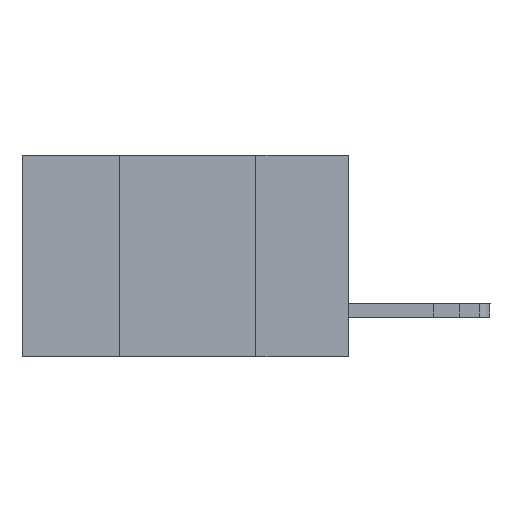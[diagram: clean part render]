
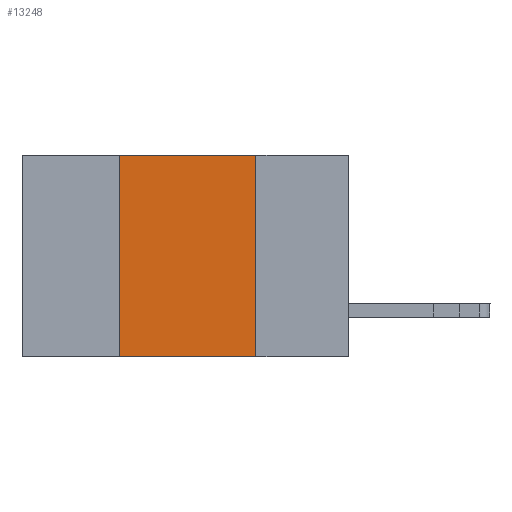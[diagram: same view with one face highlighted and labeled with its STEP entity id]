
A CAD part, left-side view. The second image highlights one B-rep face of the part: STEP entity #13248.
In plain terms, the highlighted planar face has unit normal (-1, 0, 0).
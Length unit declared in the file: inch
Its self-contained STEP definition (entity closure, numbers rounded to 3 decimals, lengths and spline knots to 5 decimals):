
#283 = VECTOR ( 'NONE', #841, 39.37008 ) ;
#434 = CARTESIAN_POINT ( 'NONE',  ( 0., 0.6, -0.37 ) ) ;
#621 = AXIS2_PLACEMENT_3D ( 'NONE', #13764, #3390, #15486 ) ;
#841 = DIRECTION ( 'NONE',  ( 0., -1., 0. ) ) ;
#1753 = VERTEX_POINT ( 'NONE', #9347 ) ;
#1844 = ORIENTED_EDGE ( 'NONE', *, *, #4746, .T. ) ;
#1912 = ORIENTED_EDGE ( 'NONE', *, *, #3890, .F. ) ;
#1971 = CARTESIAN_POINT ( 'NONE',  ( 0., 0.17, -0.37 ) ) ;
#3390 = DIRECTION ( 'NONE',  ( 1., 0., 0. ) ) ;
#3890 = EDGE_CURVE ( 'NONE', #1753, #20682, #10114, .T. ) ;
#4715 = ORIENTED_EDGE ( 'NONE', *, *, #16587, .F. ) ;
#4746 = EDGE_CURVE ( 'NONE', #8579, #16002, #18567, .T. ) ;
#5558 = LINE ( 'NONE', #10077, #14237 ) ;
#5957 = CARTESIAN_POINT ( 'NONE',  ( 0., 0.17, 0. ) ) ;
#8068 = EDGE_LOOP ( 'NONE', ( #4715, #1912, #21949, #1844 ) ) ;
#8579 = VERTEX_POINT ( 'NONE', #21644 ) ;
#9347 = CARTESIAN_POINT ( 'NONE',  ( 0., 0.42, 0. ) ) ;
#10077 = CARTESIAN_POINT ( 'NONE',  ( 0., 0.42, -0.37 ) ) ;
#10114 = LINE ( 'NONE', #14477, #14135 ) ;
#10313 = PLANE ( 'NONE',  #621 ) ;
#11211 = FACE_OUTER_BOUND ( 'NONE', #8068, .T. ) ;
#12227 = CARTESIAN_POINT ( 'NONE',  ( 0., 0.17, -0.37 ) ) ;
#13248 = ADVANCED_FACE ( 'NONE', ( #11211 ), #10313, .F. ) ;
#13764 = CARTESIAN_POINT ( 'NONE',  ( 0., 0.6, 0. ) ) ;
#13959 = DIRECTION ( 'NONE',  ( 0., -1., 0. ) ) ;
#14135 = VECTOR ( 'NONE', #13959, 39.37008 ) ;
#14237 = VECTOR ( 'NONE', #21908, 39.37008 ) ;
#14477 = CARTESIAN_POINT ( 'NONE',  ( 0., 0.6, 0. ) ) ;
#15486 = DIRECTION ( 'NONE',  ( 0., 0., -1. ) ) ;
#16002 = VERTEX_POINT ( 'NONE', #1971 ) ;
#16587 = EDGE_CURVE ( 'NONE', #20682, #16002, #21035, .T. ) ;
#16636 = VECTOR ( 'NONE', #17302, 39.37008 ) ;
#17302 = DIRECTION ( 'NONE',  ( 0., 0., -1. ) ) ;
#18567 = LINE ( 'NONE', #434, #283 ) ;
#19209 = EDGE_CURVE ( 'NONE', #8579, #1753, #5558, .T. ) ;
#20682 = VERTEX_POINT ( 'NONE', #5957 ) ;
#21035 = LINE ( 'NONE', #12227, #16636 ) ;
#21644 = CARTESIAN_POINT ( 'NONE',  ( 0., 0.42, -0.37 ) ) ;
#21908 = DIRECTION ( 'NONE',  ( 0., 0., 1. ) ) ;
#21949 = ORIENTED_EDGE ( 'NONE', *, *, #19209, .F. ) ;
